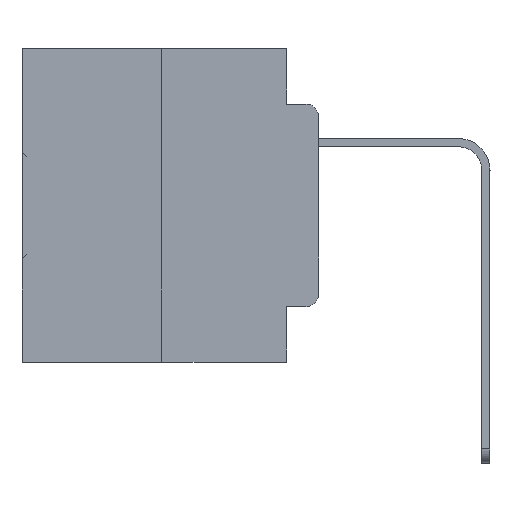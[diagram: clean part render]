
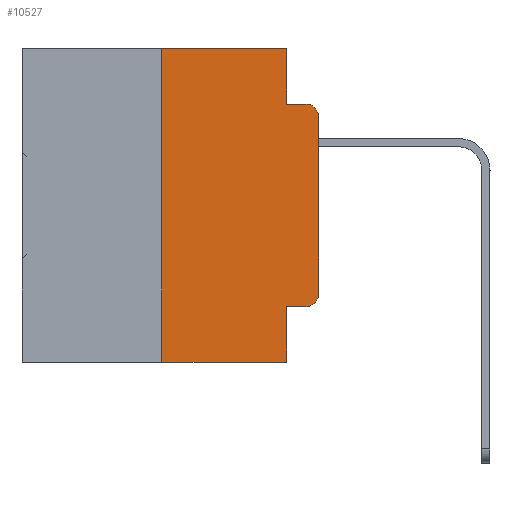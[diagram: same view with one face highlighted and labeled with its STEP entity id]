
A CAD part, left-side view. The second image highlights one B-rep face of the part: STEP entity #10527.
In plain terms, the highlighted planar face has unit normal (-1, 0, 0).
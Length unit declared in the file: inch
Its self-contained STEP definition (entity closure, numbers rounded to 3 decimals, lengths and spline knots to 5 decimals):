
#1467 = ORIENTED_EDGE ( 'NONE', *, *, #20932, .F. ) ;
#2393 = LINE ( 'NONE', #15531, #15737 ) ;
#2442 = VERTEX_POINT ( 'NONE', #12131 ) ;
#2606 = VERTEX_POINT ( 'NONE', #15726 ) ;
#2990 = DIRECTION ( 'NONE',  ( 1., 0., 0. ) ) ;
#3465 = ORIENTED_EDGE ( 'NONE', *, *, #11231, .T. ) ;
#4134 = EDGE_LOOP ( 'NONE', ( #18570, #15369, #13120, #1467, #23095, #7132, #12137, #4283, #24059, #3465 ) ) ;
#4283 = ORIENTED_EDGE ( 'NONE', *, *, #27356, .F. ) ;
#4337 = LINE ( 'NONE', #27452, #22619 ) ;
#4859 = EDGE_CURVE ( 'NONE', #4971, #21358, #29777, .T. ) ;
#4971 = VERTEX_POINT ( 'NONE', #5601 ) ;
#5420 = VERTEX_POINT ( 'NONE', #33491 ) ;
#5463 = DIRECTION ( 'NONE',  ( 0., 0., -1. ) ) ;
#5601 = CARTESIAN_POINT ( 'NONE',  ( 0., 0.051, -0.0885 ) ) ;
#5743 = CARTESIAN_POINT ( 'NONE',  ( 0., 0.25, 0. ) ) ;
#6424 = DIRECTION ( 'NONE',  ( 0., 0., 1. ) ) ;
#6656 = DIRECTION ( 'NONE',  ( 0., -1., 0. ) ) ;
#7132 = ORIENTED_EDGE ( 'NONE', *, *, #32156, .F. ) ;
#7394 = DIRECTION ( 'NONE',  ( -1., 0., 0. ) ) ;
#7919 = CIRCLE ( 'NONE', #17098, 0.02 ) ;
#8345 = CARTESIAN_POINT ( 'NONE',  ( 0., 0.473, 0. ) ) ;
#8648 = CARTESIAN_POINT ( 'NONE',  ( 0., 0., -0.3915 ) ) ;
#8670 = CARTESIAN_POINT ( 'NONE',  ( 0., 0.051, -0.4115 ) ) ;
#8753 = VECTOR ( 'NONE', #6424, 39.37008 ) ;
#10527 = ADVANCED_FACE ( 'NONE', ( #14084 ), #30120, .F. ) ;
#10591 = EDGE_CURVE ( 'NONE', #23924, #5420, #29383, .T. ) ;
#10676 = LINE ( 'NONE', #8670, #15261 ) ;
#10779 = DIRECTION ( 'NONE',  ( -1., 0., 0. ) ) ;
#10919 = EDGE_CURVE ( 'NONE', #14878, #13225, #2393, .T. ) ;
#11231 = EDGE_CURVE ( 'NONE', #2442, #14878, #25646, .T. ) ;
#11253 = CARTESIAN_POINT ( 'NONE',  ( 0., 0.473, -0.5 ) ) ;
#11399 = EDGE_CURVE ( 'NONE', #14527, #2442, #10676, .T. ) ;
#11848 = DIRECTION ( 'NONE',  ( 0., -1., 0. ) ) ;
#12131 = CARTESIAN_POINT ( 'NONE',  ( 0., 0.02, -0.4115 ) ) ;
#12137 = ORIENTED_EDGE ( 'NONE', *, *, #30402, .T. ) ;
#12699 = CARTESIAN_POINT ( 'NONE',  ( 0., 0.051, -0.5 ) ) ;
#13120 = ORIENTED_EDGE ( 'NONE', *, *, #4859, .F. ) ;
#13225 = VERTEX_POINT ( 'NONE', #23050 ) ;
#14084 = FACE_OUTER_BOUND ( 'NONE', #4134, .T. ) ;
#14368 = DIRECTION ( 'NONE',  ( 0., 0., -1. ) ) ;
#14527 = VERTEX_POINT ( 'NONE', #28717 ) ;
#14878 = VERTEX_POINT ( 'NONE', #8648 ) ;
#15261 = VECTOR ( 'NONE', #24579, 39.37008 ) ;
#15369 = ORIENTED_EDGE ( 'NONE', *, *, #23493, .T. ) ;
#15531 = CARTESIAN_POINT ( 'NONE',  ( 0., 0., 0. ) ) ;
#15684 = VECTOR ( 'NONE', #22172, 39.37008 ) ;
#15726 = CARTESIAN_POINT ( 'NONE',  ( 0., 0.25, -0.5 ) ) ;
#15737 = VECTOR ( 'NONE', #28807, 39.37008 ) ;
#17098 = AXIS2_PLACEMENT_3D ( 'NONE', #28499, #7394, #20757 ) ;
#18570 = ORIENTED_EDGE ( 'NONE', *, *, #10919, .T. ) ;
#19751 = CARTESIAN_POINT ( 'NONE',  ( 0., 0.473, 0. ) ) ;
#20009 = VERTEX_POINT ( 'NONE', #12699 ) ;
#20757 = DIRECTION ( 'NONE',  ( 0., 0., -1. ) ) ;
#20842 = AXIS2_PLACEMENT_3D ( 'NONE', #19751, #2990, #5463 ) ;
#20932 = EDGE_CURVE ( 'NONE', #5420, #4971, #4337, .T. ) ;
#21358 = VERTEX_POINT ( 'NONE', #28932 ) ;
#22172 = DIRECTION ( 'NONE',  ( 0., -1., 0. ) ) ;
#22619 = VECTOR ( 'NONE', #14368, 39.37008 ) ;
#23050 = CARTESIAN_POINT ( 'NONE',  ( 0., 0., -0.1085 ) ) ;
#23095 = ORIENTED_EDGE ( 'NONE', *, *, #10591, .F. ) ;
#23344 = VECTOR ( 'NONE', #27838, 39.37008 ) ;
#23493 = EDGE_CURVE ( 'NONE', #13225, #21358, #7919, .T. ) ;
#23924 = VERTEX_POINT ( 'NONE', #32863 ) ;
#24059 = ORIENTED_EDGE ( 'NONE', *, *, #11399, .T. ) ;
#24579 = DIRECTION ( 'NONE',  ( 0., -1., 0. ) ) ;
#25150 = CARTESIAN_POINT ( 'NONE',  ( 0., 0.051, -0.0885 ) ) ;
#25278 = VECTOR ( 'NONE', #6656, 39.37008 ) ;
#25646 = CIRCLE ( 'NONE', #33036, 0.02 ) ;
#27356 = EDGE_CURVE ( 'NONE', #14527, #20009, #32010, .T. ) ;
#27452 = CARTESIAN_POINT ( 'NONE',  ( 0., 0.051, 0. ) ) ;
#27604 = CARTESIAN_POINT ( 'NONE',  ( 0., 0.051, 0. ) ) ;
#27838 = DIRECTION ( 'NONE',  ( 0., 0., -1. ) ) ;
#28499 = CARTESIAN_POINT ( 'NONE',  ( 0., 0.02, -0.1085 ) ) ;
#28717 = CARTESIAN_POINT ( 'NONE',  ( 0., 0.051, -0.4115 ) ) ;
#28807 = DIRECTION ( 'NONE',  ( 0., 0., 1. ) ) ;
#28932 = CARTESIAN_POINT ( 'NONE',  ( 0., 0.02, -0.0885 ) ) ;
#29383 = LINE ( 'NONE', #8345, #30195 ) ;
#29777 = LINE ( 'NONE', #25150, #25278 ) ;
#29890 = LINE ( 'NONE', #5743, #8753 ) ;
#30120 = PLANE ( 'NONE',  #20842 ) ;
#30195 = VECTOR ( 'NONE', #11848, 39.37008 ) ;
#30402 = EDGE_CURVE ( 'NONE', #2606, #20009, #32222, .T. ) ;
#31962 = CARTESIAN_POINT ( 'NONE',  ( 0., 0.02, -0.3915 ) ) ;
#32010 = LINE ( 'NONE', #27604, #23344 ) ;
#32076 = DIRECTION ( 'NONE',  ( 0., 0., -1. ) ) ;
#32156 = EDGE_CURVE ( 'NONE', #2606, #23924, #29890, .T. ) ;
#32222 = LINE ( 'NONE', #11253, #15684 ) ;
#32863 = CARTESIAN_POINT ( 'NONE',  ( 0., 0.25, 0. ) ) ;
#33036 = AXIS2_PLACEMENT_3D ( 'NONE', #31962, #10779, #32076 ) ;
#33491 = CARTESIAN_POINT ( 'NONE',  ( 0., 0.051, 0. ) ) ;
